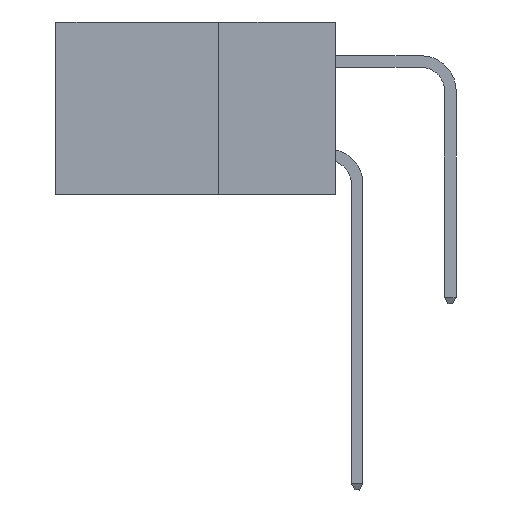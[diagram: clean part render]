
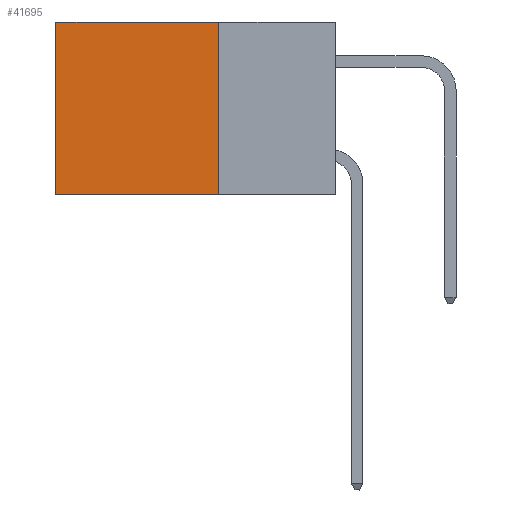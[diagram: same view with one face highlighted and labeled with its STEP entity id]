
A CAD part, left-side view. The second image highlights one B-rep face of the part: STEP entity #41695.
In plain terms, the highlighted planar face has unit normal (-1, 0, 0).
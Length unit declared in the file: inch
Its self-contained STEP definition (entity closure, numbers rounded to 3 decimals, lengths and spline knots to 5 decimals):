
#146 = PLANE ( 'NONE',  #21221 ) ;
#1417 = VERTEX_POINT ( 'NONE', #20639 ) ;
#3914 = LINE ( 'NONE', #17575, #13252 ) ;
#6043 = DIRECTION ( 'NONE',  ( 0., 1., 0. ) ) ;
#6227 = EDGE_CURVE ( 'NONE', #1417, #36134, #23033, .T. ) ;
#7160 = ORIENTED_EDGE ( 'NONE', *, *, #13472, .T. ) ;
#7865 = ORIENTED_EDGE ( 'NONE', *, *, #16243, .T. ) ;
#9238 = VECTOR ( 'NONE', #11131, 39.37008 ) ;
#11126 = DIRECTION ( 'NONE',  ( 1., 0., 0. ) ) ;
#11131 = DIRECTION ( 'NONE',  ( 0., 1., 0. ) ) ;
#12753 = CARTESIAN_POINT ( 'NONE',  ( 0.2875, 0.6, -0.37 ) ) ;
#13252 = VECTOR ( 'NONE', #31199, 39.37008 ) ;
#13472 = EDGE_CURVE ( 'NONE', #16983, #15988, #38375, .T. ) ;
#14256 = FACE_OUTER_BOUND ( 'NONE', #25492, .T. ) ;
#14653 = CARTESIAN_POINT ( 'NONE',  ( 0.2875, 0.25, 0. ) ) ;
#15004 = VECTOR ( 'NONE', #6043, 39.37008 ) ;
#15988 = VERTEX_POINT ( 'NONE', #36497 ) ;
#16243 = EDGE_CURVE ( 'NONE', #15988, #36134, #25899, .T. ) ;
#16983 = VERTEX_POINT ( 'NONE', #14653 ) ;
#17182 = CARTESIAN_POINT ( 'NONE',  ( 0.2875, 0.25, 0. ) ) ;
#17575 = CARTESIAN_POINT ( 'NONE',  ( 0.2875, 0.25, 0. ) ) ;
#18518 = ORIENTED_EDGE ( 'NONE', *, *, #6227, .F. ) ;
#20639 = CARTESIAN_POINT ( 'NONE',  ( 0.2875, 0.25, -0.37 ) ) ;
#21221 = AXIS2_PLACEMENT_3D ( 'NONE', #31238, #11126, #41500 ) ;
#23033 = LINE ( 'NONE', #36677, #15004 ) ;
#25492 = EDGE_LOOP ( 'NONE', ( #7865, #18518, #41902, #7160 ) ) ;
#25666 = EDGE_CURVE ( 'NONE', #16983, #1417, #3914, .T. ) ;
#25899 = LINE ( 'NONE', #35752, #39449 ) ;
#31199 = DIRECTION ( 'NONE',  ( 0., 0., -1. ) ) ;
#31238 = CARTESIAN_POINT ( 'NONE',  ( 0.2875, 0.25, 0. ) ) ;
#35752 = CARTESIAN_POINT ( 'NONE',  ( 0.2875, 0.6, 0. ) ) ;
#36134 = VERTEX_POINT ( 'NONE', #12753 ) ;
#36403 = DIRECTION ( 'NONE',  ( 0., 0., -1. ) ) ;
#36497 = CARTESIAN_POINT ( 'NONE',  ( 0.2875, 0.6, 0. ) ) ;
#36677 = CARTESIAN_POINT ( 'NONE',  ( 0.2875, 0.25, -0.37 ) ) ;
#38375 = LINE ( 'NONE', #17182, #9238 ) ;
#39449 = VECTOR ( 'NONE', #36403, 39.37008 ) ;
#41500 = DIRECTION ( 'NONE',  ( 0., 0., -1. ) ) ;
#41695 = ADVANCED_FACE ( 'NONE', ( #14256 ), #146, .F. ) ;
#41902 = ORIENTED_EDGE ( 'NONE', *, *, #25666, .F. ) ;
